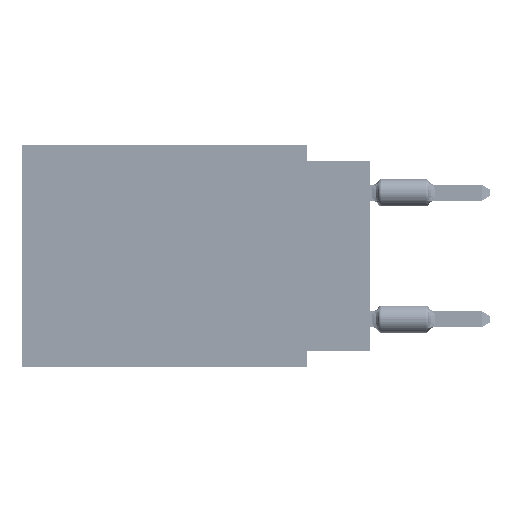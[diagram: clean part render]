
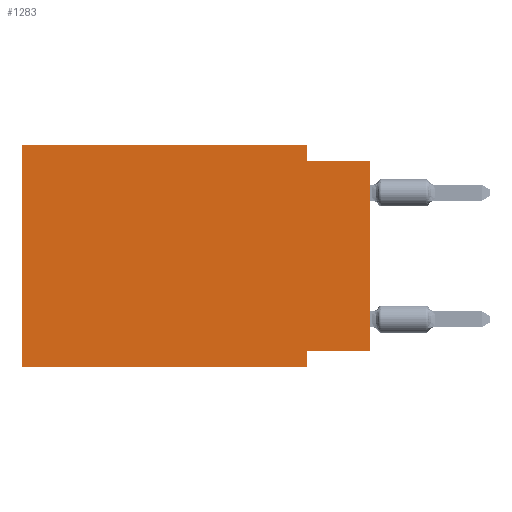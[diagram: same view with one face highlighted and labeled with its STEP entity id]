
A CAD part, left-side view. The second image highlights one B-rep face of the part: STEP entity #1283.
In plain terms, the highlighted planar face has unit normal (-1, 0, 0).
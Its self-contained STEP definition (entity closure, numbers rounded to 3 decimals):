
#1283 = ADVANCED_FACE ( 'NONE', ( #1814 ), #86817, .F. ) ;
#1814 = FACE_OUTER_BOUND ( 'NONE', #89231, .T. ) ;
#2283 = ORIENTED_EDGE ( 'NONE', *, *, #47861, .T. ) ;
#3865 = CARTESIAN_POINT ( 'NONE',  ( 0., 2.54, -8.89 ) ) ;
#6607 = LINE ( 'NONE', #33227, #84130 ) ;
#7553 = EDGE_CURVE ( 'NONE', #74526, #28610, #31055, .T. ) ;
#9775 = EDGE_CURVE ( 'NONE', #69744, #73113, #6607, .T. ) ;
#12194 = DIRECTION ( 'NONE',  ( 0., 0., 1. ) ) ;
#15194 = CARTESIAN_POINT ( 'NONE',  ( 0., 13.97, 0. ) ) ;
#16548 = DIRECTION ( 'NONE',  ( 0., -1., 0. ) ) ;
#17310 = DIRECTION ( 'NONE',  ( 0., -1., 0. ) ) ;
#17790 = ORIENTED_EDGE ( 'NONE', *, *, #50604, .T. ) ;
#18580 = VERTEX_POINT ( 'NONE', #90647 ) ;
#18815 = ORIENTED_EDGE ( 'NONE', *, *, #7553, .F. ) ;
#19366 = VERTEX_POINT ( 'NONE', #59476 ) ;
#22356 = DIRECTION ( 'NONE',  ( 0., 0., -1. ) ) ;
#22715 = CARTESIAN_POINT ( 'NONE',  ( 0., 2.54, -8.255 ) ) ;
#23372 = CARTESIAN_POINT ( 'NONE',  ( 0., 2.54, 0. ) ) ;
#23593 = VERTEX_POINT ( 'NONE', #68933 ) ;
#23737 = DIRECTION ( 'NONE',  ( 1., 0., 0. ) ) ;
#25558 = ORIENTED_EDGE ( 'NONE', *, *, #55519, .F. ) ;
#27139 = DIRECTION ( 'NONE',  ( 0., 0., -1. ) ) ;
#28208 = EDGE_CURVE ( 'NONE', #28610, #18580, #29908, .T. ) ;
#28610 = VERTEX_POINT ( 'NONE', #37620 ) ;
#28905 = CARTESIAN_POINT ( 'NONE',  ( 0., 13.97, 0. ) ) ;
#29908 = LINE ( 'NONE', #23372, #39662 ) ;
#31014 = LINE ( 'NONE', #80101, #84478 ) ;
#31055 = LINE ( 'NONE', #15194, #37641 ) ;
#33204 = CARTESIAN_POINT ( 'NONE',  ( 0., 0., 0. ) ) ;
#33227 = CARTESIAN_POINT ( 'NONE',  ( 0., 2.54, -8.89 ) ) ;
#34644 = CARTESIAN_POINT ( 'NONE',  ( 0., 13.97, 0. ) ) ;
#37620 = CARTESIAN_POINT ( 'NONE',  ( 0., 2.54, 0. ) ) ;
#37641 = VECTOR ( 'NONE', #81056, 1000. ) ;
#38725 = CARTESIAN_POINT ( 'NONE',  ( 0., 13.97, 0. ) ) ;
#39289 = VECTOR ( 'NONE', #17310, 1000. ) ;
#39662 = VECTOR ( 'NONE', #43008, 1000. ) ;
#43008 = DIRECTION ( 'NONE',  ( 0., 0., -1. ) ) ;
#43892 = VECTOR ( 'NONE', #53227, 1000. ) ;
#45862 = LINE ( 'NONE', #33204, #64993 ) ;
#47861 = EDGE_CURVE ( 'NONE', #19366, #73113, #88782, .T. ) ;
#50464 = ORIENTED_EDGE ( 'NONE', *, *, #28208, .F. ) ;
#50604 = EDGE_CURVE ( 'NONE', #51689, #23593, #45862, .T. ) ;
#51517 = CARTESIAN_POINT ( 'NONE',  ( 0., 0., -8.255 ) ) ;
#51689 = VERTEX_POINT ( 'NONE', #51517 ) ;
#52133 = ORIENTED_EDGE ( 'NONE', *, *, #85568, .F. ) ;
#53227 = DIRECTION ( 'NONE',  ( 0., 0., 1. ) ) ;
#53339 = LINE ( 'NONE', #81818, #84531 ) ;
#54954 = ORIENTED_EDGE ( 'NONE', *, *, #86147, .F. ) ;
#55519 = EDGE_CURVE ( 'NONE', #19366, #74526, #60679, .T. ) ;
#57789 = AXIS2_PLACEMENT_3D ( 'NONE', #28905, #23737, #22356 ) ;
#57999 = ORIENTED_EDGE ( 'NONE', *, *, #9775, .F. ) ;
#59476 = CARTESIAN_POINT ( 'NONE',  ( 0., 13.97, -8.89 ) ) ;
#60679 = LINE ( 'NONE', #38725, #43892 ) ;
#61241 = DIRECTION ( 'NONE',  ( 0., 1., 0. ) ) ;
#64993 = VECTOR ( 'NONE', #12194, 1000. ) ;
#68933 = CARTESIAN_POINT ( 'NONE',  ( 0., 0., -0.635 ) ) ;
#69744 = VERTEX_POINT ( 'NONE', #22715 ) ;
#73113 = VERTEX_POINT ( 'NONE', #3865 ) ;
#74526 = VERTEX_POINT ( 'NONE', #34644 ) ;
#80101 = CARTESIAN_POINT ( 'NONE',  ( 0., 0., -0.635 ) ) ;
#81056 = DIRECTION ( 'NONE',  ( 0., -1., 0. ) ) ;
#81818 = CARTESIAN_POINT ( 'NONE',  ( 0., 0., -8.255 ) ) ;
#84130 = VECTOR ( 'NONE', #27139, 1000. ) ;
#84478 = VECTOR ( 'NONE', #16548, 1000. ) ;
#84531 = VECTOR ( 'NONE', #61241, 1000. ) ;
#85568 = EDGE_CURVE ( 'NONE', #18580, #23593, #31014, .T. ) ;
#86147 = EDGE_CURVE ( 'NONE', #51689, #69744, #53339, .T. ) ;
#86817 = PLANE ( 'NONE',  #57789 ) ;
#88324 = CARTESIAN_POINT ( 'NONE',  ( 0., 13.97, -8.89 ) ) ;
#88782 = LINE ( 'NONE', #88324, #39289 ) ;
#89231 = EDGE_LOOP ( 'NONE', ( #17790, #52133, #50464, #18815, #25558, #2283, #57999, #54954 ) ) ;
#90647 = CARTESIAN_POINT ( 'NONE',  ( 0., 2.54, -0.635 ) ) ;
